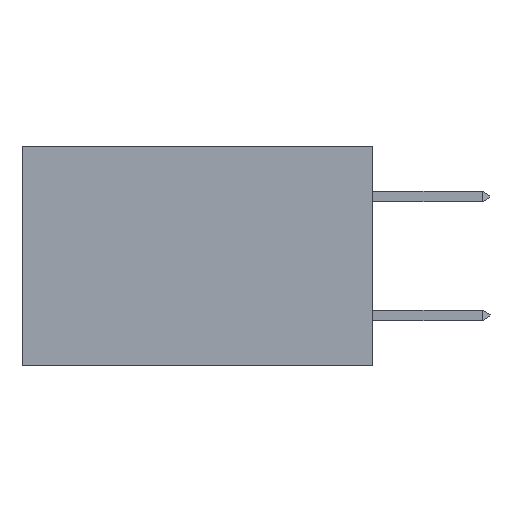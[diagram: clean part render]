
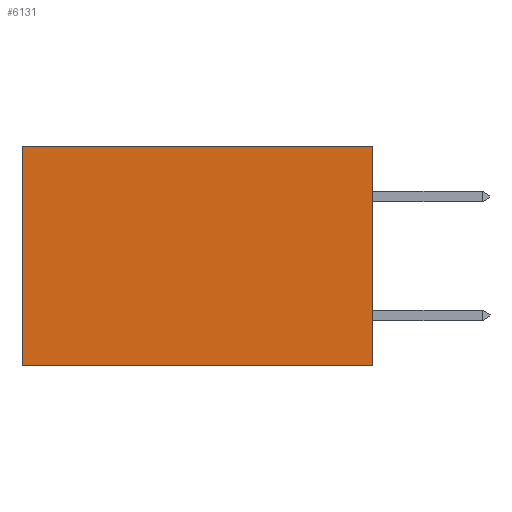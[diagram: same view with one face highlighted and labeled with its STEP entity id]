
A CAD part, left-side view. The second image highlights one B-rep face of the part: STEP entity #6131.
In plain terms, the highlighted planar face has unit normal (-1, 0, 0).
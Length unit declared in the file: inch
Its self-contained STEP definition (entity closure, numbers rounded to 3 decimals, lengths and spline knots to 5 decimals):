
#254 = CARTESIAN_POINT ( 'NONE',  ( 0.277, 0.59, -0.37 ) ) ;
#603 = CARTESIAN_POINT ( 'NONE',  ( 0.277, 0., -0.37 ) ) ;
#674 = CARTESIAN_POINT ( 'NONE',  ( 0.277, 0.59, -0.37 ) ) ;
#1163 = AXIS2_PLACEMENT_3D ( 'NONE', #4785, #7003, #21442 ) ;
#1186 = FACE_OUTER_BOUND ( 'NONE', #13251, .T. ) ;
#1891 = VERTEX_POINT ( 'NONE', #254 ) ;
#2680 = DIRECTION ( 'NONE',  ( 0., 1., 0. ) ) ;
#4785 = CARTESIAN_POINT ( 'NONE',  ( 0.277, 0., -0.37 ) ) ;
#5358 = DIRECTION ( 'NONE',  ( 0., 0., -1. ) ) ;
#6131 = ADVANCED_FACE ( 'NONE', ( #1186 ), #19379, .F. ) ;
#6992 = VECTOR ( 'NONE', #2680, 39.37008 ) ;
#7003 = DIRECTION ( 'NONE',  ( 1., 0., 0. ) ) ;
#7267 = ORIENTED_EDGE ( 'NONE', *, *, #18387, .F. ) ;
#7648 = LINE ( 'NONE', #603, #6992 ) ;
#8793 = CARTESIAN_POINT ( 'NONE',  ( 0.277, 0., 0. ) ) ;
#9321 = DIRECTION ( 'NONE',  ( 0., 1., 0. ) ) ;
#9828 = DIRECTION ( 'NONE',  ( 0., 0., -1. ) ) ;
#11122 = EDGE_CURVE ( 'NONE', #19412, #22886, #21991, .T. ) ;
#12488 = LINE ( 'NONE', #674, #22145 ) ;
#12940 = ORIENTED_EDGE ( 'NONE', *, *, #21398, .F. ) ;
#13059 = CARTESIAN_POINT ( 'NONE',  ( 0.277, 0.59, 0. ) ) ;
#13251 = EDGE_LOOP ( 'NONE', ( #21180, #12940, #7267, #18139 ) ) ;
#13988 = CARTESIAN_POINT ( 'NONE',  ( 0.277, 0., -0.37 ) ) ;
#14024 = EDGE_CURVE ( 'NONE', #22886, #1891, #12488, .T. ) ;
#14096 = VERTEX_POINT ( 'NONE', #17869 ) ;
#17869 = CARTESIAN_POINT ( 'NONE',  ( 0.277, 0., -0.37 ) ) ;
#18139 = ORIENTED_EDGE ( 'NONE', *, *, #11122, .T. ) ;
#18387 = EDGE_CURVE ( 'NONE', #19412, #14096, #25831, .T. ) ;
#19379 = PLANE ( 'NONE',  #1163 ) ;
#19412 = VERTEX_POINT ( 'NONE', #8793 ) ;
#20408 = VECTOR ( 'NONE', #9828, 39.37008 ) ;
#21180 = ORIENTED_EDGE ( 'NONE', *, *, #14024, .T. ) ;
#21336 = VECTOR ( 'NONE', #9321, 39.37008 ) ;
#21398 = EDGE_CURVE ( 'NONE', #14096, #1891, #7648, .T. ) ;
#21442 = DIRECTION ( 'NONE',  ( 0., 0., -1. ) ) ;
#21991 = LINE ( 'NONE', #23699, #21336 ) ;
#22145 = VECTOR ( 'NONE', #5358, 39.37008 ) ;
#22886 = VERTEX_POINT ( 'NONE', #13059 ) ;
#23699 = CARTESIAN_POINT ( 'NONE',  ( 0.277, 0., 0. ) ) ;
#25831 = LINE ( 'NONE', #13988, #20408 ) ;
